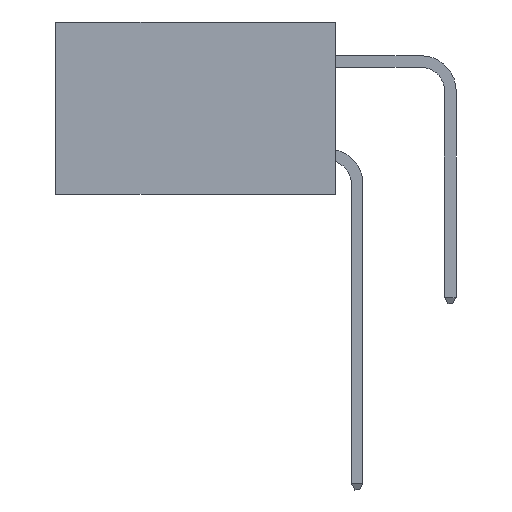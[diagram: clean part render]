
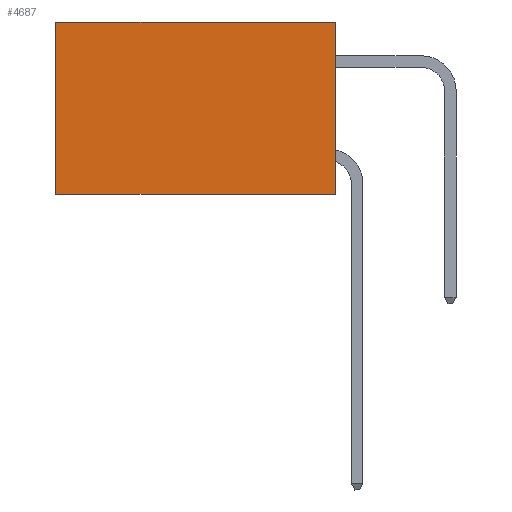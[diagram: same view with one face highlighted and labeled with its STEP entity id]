
A CAD part, left-side view. The second image highlights one B-rep face of the part: STEP entity #4687.
In plain terms, the highlighted planar face has unit normal (-1, 0, 0).
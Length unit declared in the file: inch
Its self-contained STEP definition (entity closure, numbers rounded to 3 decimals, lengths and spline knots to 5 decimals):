
#5 = VERTEX_POINT ( 'NONE', #28943 ) ;
#409 = CARTESIAN_POINT ( 'NONE',  ( 0.2875, 0.6, -0.37 ) ) ;
#1838 = CARTESIAN_POINT ( 'NONE',  ( 0.2875, 0.6, 0. ) ) ;
#1975 = DIRECTION ( 'NONE',  ( 0., 1., 0. ) ) ;
#2278 = LINE ( 'NONE', #7682, #5662 ) ;
#2837 = ORIENTED_EDGE ( 'NONE', *, *, #26731, .T. ) ;
#4625 = EDGE_CURVE ( 'NONE', #5, #8344, #11922, .T. ) ;
#4687 = ADVANCED_FACE ( 'NONE', ( #10361 ), #25670, .F. ) ;
#5209 = EDGE_CURVE ( 'NONE', #29067, #30200, #8849, .T. ) ;
#5662 = VECTOR ( 'NONE', #22823, 39.37008 ) ;
#7682 = CARTESIAN_POINT ( 'NONE',  ( 0.2875, 0., -0.37 ) ) ;
#8344 = VERTEX_POINT ( 'NONE', #27153 ) ;
#8849 = LINE ( 'NONE', #1838, #19967 ) ;
#10361 = FACE_OUTER_BOUND ( 'NONE', #11895, .T. ) ;
#11895 = EDGE_LOOP ( 'NONE', ( #13272, #30610, #19238, #2837 ) ) ;
#11922 = LINE ( 'NONE', #30154, #15713 ) ;
#11986 = DIRECTION ( 'NONE',  ( 0., 0., -1. ) ) ;
#13272 = ORIENTED_EDGE ( 'NONE', *, *, #5209, .T. ) ;
#15130 = DIRECTION ( 'NONE',  ( 0., 0., -1. ) ) ;
#15713 = VECTOR ( 'NONE', #15130, 39.37008 ) ;
#15989 = CARTESIAN_POINT ( 'NONE',  ( 0.2875, 0., 0. ) ) ;
#16847 = CARTESIAN_POINT ( 'NONE',  ( 0.2875, 0., 0. ) ) ;
#17577 = CARTESIAN_POINT ( 'NONE',  ( 0.2875, 0.6, 0. ) ) ;
#18348 = DIRECTION ( 'NONE',  ( 0., 0., -1. ) ) ;
#19079 = LINE ( 'NONE', #16847, #19838 ) ;
#19238 = ORIENTED_EDGE ( 'NONE', *, *, #4625, .F. ) ;
#19838 = VECTOR ( 'NONE', #1975, 39.37008 ) ;
#19967 = VECTOR ( 'NONE', #11986, 39.37008 ) ;
#20917 = DIRECTION ( 'NONE',  ( 1., 0., 0. ) ) ;
#22823 = DIRECTION ( 'NONE',  ( 0., 1., 0. ) ) ;
#25657 = AXIS2_PLACEMENT_3D ( 'NONE', #15989, #20917, #18348 ) ;
#25670 = PLANE ( 'NONE',  #25657 ) ;
#26333 = EDGE_CURVE ( 'NONE', #8344, #30200, #2278, .T. ) ;
#26731 = EDGE_CURVE ( 'NONE', #5, #29067, #19079, .T. ) ;
#27153 = CARTESIAN_POINT ( 'NONE',  ( 0.2875, 0., -0.37 ) ) ;
#28943 = CARTESIAN_POINT ( 'NONE',  ( 0.2875, 0., 0. ) ) ;
#29067 = VERTEX_POINT ( 'NONE', #17577 ) ;
#30154 = CARTESIAN_POINT ( 'NONE',  ( 0.2875, 0., 0. ) ) ;
#30200 = VERTEX_POINT ( 'NONE', #409 ) ;
#30610 = ORIENTED_EDGE ( 'NONE', *, *, #26333, .F. ) ;
